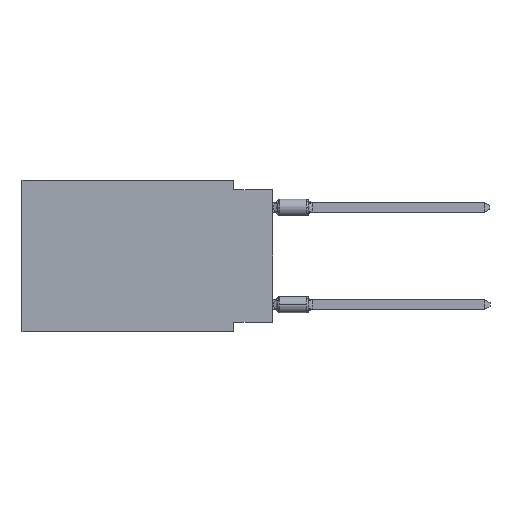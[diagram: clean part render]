
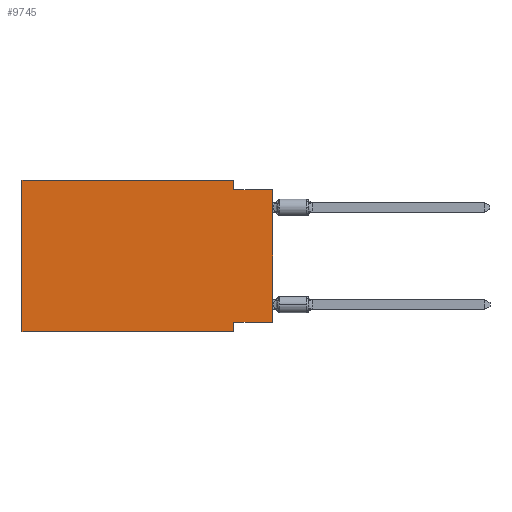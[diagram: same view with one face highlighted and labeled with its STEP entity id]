
A CAD part, left-side view. The second image highlights one B-rep face of the part: STEP entity #9745.
In plain terms, the highlighted planar face has unit normal (-1, 0, 0).
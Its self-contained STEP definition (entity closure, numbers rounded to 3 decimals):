
#23 = CARTESIAN_POINT ( 'NONE',  ( 0., 2.54, -0.635 ) ) ;
#794 = LINE ( 'NONE', #13407, #5103 ) ;
#1352 = VERTEX_POINT ( 'NONE', #13899 ) ;
#2190 = CARTESIAN_POINT ( 'NONE',  ( 0., 16.383, -9.906 ) ) ;
#2510 = CARTESIAN_POINT ( 'NONE',  ( 0., 0., -0.635 ) ) ;
#2798 = DIRECTION ( 'NONE',  ( 0., 1., 0. ) ) ;
#3147 = DIRECTION ( 'NONE',  ( 0., 0., -1. ) ) ;
#3203 = ORIENTED_EDGE ( 'NONE', *, *, #10358, .F. ) ;
#3267 = ORIENTED_EDGE ( 'NONE', *, *, #16404, .F. ) ;
#4931 = CARTESIAN_POINT ( 'NONE',  ( 0., 2.54, -9.906 ) ) ;
#4939 = ORIENTED_EDGE ( 'NONE', *, *, #5025, .F. ) ;
#5025 = EDGE_CURVE ( 'NONE', #15855, #9114, #5814, .T. ) ;
#5103 = VECTOR ( 'NONE', #6946, 1000. ) ;
#5456 = LINE ( 'NONE', #16564, #13830 ) ;
#5658 = CARTESIAN_POINT ( 'NONE',  ( 0., 0., -9.271 ) ) ;
#5756 = VERTEX_POINT ( 'NONE', #5658 ) ;
#5814 = LINE ( 'NONE', #2510, #14590 ) ;
#5896 = VERTEX_POINT ( 'NONE', #12214 ) ;
#6020 = ORIENTED_EDGE ( 'NONE', *, *, #6166, .F. ) ;
#6166 = EDGE_CURVE ( 'NONE', #5756, #7062, #7245, .T. ) ;
#6946 = DIRECTION ( 'NONE',  ( 0., -1., 0. ) ) ;
#7062 = VERTEX_POINT ( 'NONE', #12865 ) ;
#7167 = DIRECTION ( 'NONE',  ( 0., -1., 0. ) ) ;
#7245 = LINE ( 'NONE', #17958, #15670 ) ;
#7490 = VECTOR ( 'NONE', #3147, 1000. ) ;
#8384 = VECTOR ( 'NONE', #17213, 1000. ) ;
#8411 = DIRECTION ( 'NONE',  ( 0., 0., -1. ) ) ;
#8464 = LINE ( 'NONE', #13215, #9338 ) ;
#8503 = CARTESIAN_POINT ( 'NONE',  ( 0., 16.383, 0. ) ) ;
#9114 = VERTEX_POINT ( 'NONE', #13398 ) ;
#9338 = VECTOR ( 'NONE', #13016, 1000. ) ;
#9587 = ORIENTED_EDGE ( 'NONE', *, *, #17258, .T. ) ;
#9636 = VECTOR ( 'NONE', #11093, 1000. ) ;
#9644 = DIRECTION ( 'NONE',  ( 1., 0., 0. ) ) ;
#9745 = ADVANCED_FACE ( 'NONE', ( #16094 ), #19015, .F. ) ;
#10358 = EDGE_CURVE ( 'NONE', #14720, #15855, #18493, .T. ) ;
#11045 = CARTESIAN_POINT ( 'NONE',  ( 0., 16.383, 0. ) ) ;
#11093 = DIRECTION ( 'NONE',  ( 0., 0., -1. ) ) ;
#12214 = CARTESIAN_POINT ( 'NONE',  ( 0., 2.54, -9.906 ) ) ;
#12865 = CARTESIAN_POINT ( 'NONE',  ( 0., 2.54, -9.271 ) ) ;
#13016 = DIRECTION ( 'NONE',  ( 0., 0., 1. ) ) ;
#13215 = CARTESIAN_POINT ( 'NONE',  ( 0., 0., 0. ) ) ;
#13398 = CARTESIAN_POINT ( 'NONE',  ( 0., 0., -0.635 ) ) ;
#13407 = CARTESIAN_POINT ( 'NONE',  ( 0., 16.383, 0. ) ) ;
#13830 = VECTOR ( 'NONE', #7167, 1000. ) ;
#13899 = CARTESIAN_POINT ( 'NONE',  ( 0., 16.383, 0. ) ) ;
#14265 = VERTEX_POINT ( 'NONE', #2190 ) ;
#14590 = VECTOR ( 'NONE', #14907, 1000. ) ;
#14720 = VERTEX_POINT ( 'NONE', #17407 ) ;
#14907 = DIRECTION ( 'NONE',  ( 0., -1., 0. ) ) ;
#15168 = CARTESIAN_POINT ( 'NONE',  ( 0., 2.54, 0. ) ) ;
#15670 = VECTOR ( 'NONE', #2798, 1000. ) ;
#15855 = VERTEX_POINT ( 'NONE', #23 ) ;
#16094 = FACE_OUTER_BOUND ( 'NONE', #16226, .T. ) ;
#16226 = EDGE_LOOP ( 'NONE', ( #17715, #4939, #3203, #3267, #16749, #9587, #16272, #6020 ) ) ;
#16272 = ORIENTED_EDGE ( 'NONE', *, *, #16294, .F. ) ;
#16294 = EDGE_CURVE ( 'NONE', #7062, #5896, #18765, .T. ) ;
#16404 = EDGE_CURVE ( 'NONE', #1352, #14720, #794, .T. ) ;
#16564 = CARTESIAN_POINT ( 'NONE',  ( 0., 16.383, -9.906 ) ) ;
#16749 = ORIENTED_EDGE ( 'NONE', *, *, #18384, .F. ) ;
#17213 = DIRECTION ( 'NONE',  ( 0., 0., 1. ) ) ;
#17258 = EDGE_CURVE ( 'NONE', #14265, #5896, #5456, .T. ) ;
#17320 = LINE ( 'NONE', #11045, #8384 ) ;
#17407 = CARTESIAN_POINT ( 'NONE',  ( 0., 2.54, 0. ) ) ;
#17611 = EDGE_CURVE ( 'NONE', #5756, #9114, #8464, .T. ) ;
#17715 = ORIENTED_EDGE ( 'NONE', *, *, #17611, .T. ) ;
#17811 = AXIS2_PLACEMENT_3D ( 'NONE', #8503, #9644, #8411 ) ;
#17958 = CARTESIAN_POINT ( 'NONE',  ( 0., 0., -9.271 ) ) ;
#18384 = EDGE_CURVE ( 'NONE', #14265, #1352, #17320, .T. ) ;
#18493 = LINE ( 'NONE', #15168, #7490 ) ;
#18765 = LINE ( 'NONE', #4931, #9636 ) ;
#19015 = PLANE ( 'NONE',  #17811 ) ;
